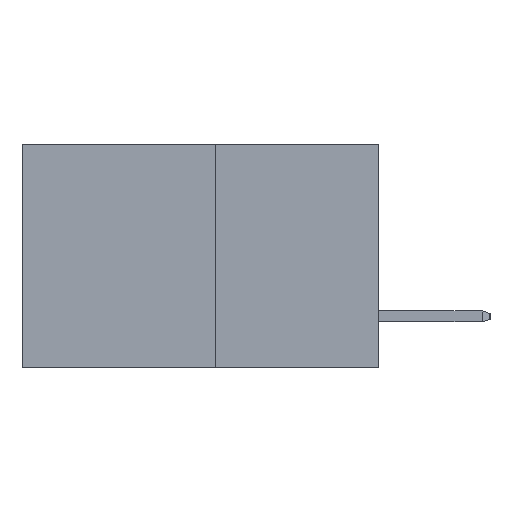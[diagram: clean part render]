
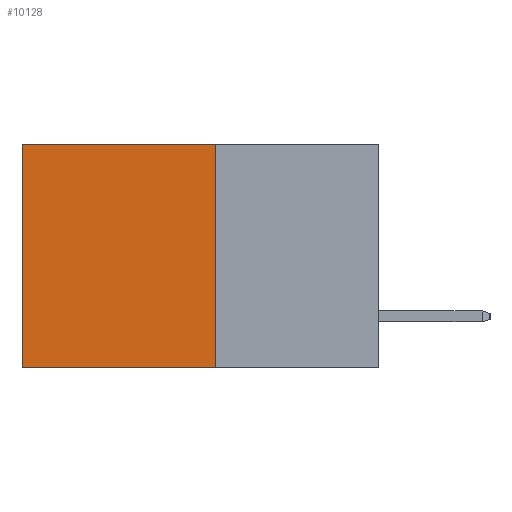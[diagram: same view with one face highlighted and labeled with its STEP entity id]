
A CAD part, left-side view. The second image highlights one B-rep face of the part: STEP entity #10128.
In plain terms, the highlighted planar face has unit normal (-1, 0, 0).
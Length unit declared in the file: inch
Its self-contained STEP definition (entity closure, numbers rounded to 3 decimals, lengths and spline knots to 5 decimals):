
#259 = ORIENTED_EDGE ( 'NONE', *, *, #10974, .T. ) ;
#437 = DIRECTION ( 'NONE',  ( 1., 0., 0. ) ) ;
#1027 = VERTEX_POINT ( 'NONE', #2424 ) ;
#1223 = ORIENTED_EDGE ( 'NONE', *, *, #10586, .F. ) ;
#1614 = ORIENTED_EDGE ( 'NONE', *, *, #4068, .F. ) ;
#2012 = VECTOR ( 'NONE', #6748, 39.37008 ) ;
#2424 = CARTESIAN_POINT ( 'NONE',  ( 0.277, 0.59, 0. ) ) ;
#2429 = CARTESIAN_POINT ( 'NONE',  ( 0.277, 0.59, -0.37 ) ) ;
#2477 = CARTESIAN_POINT ( 'NONE',  ( 0.277, 0.27, -0.37 ) ) ;
#3446 = LINE ( 'NONE', #11366, #6398 ) ;
#3470 = CARTESIAN_POINT ( 'NONE',  ( 0.277, 0.27, -0.37 ) ) ;
#3932 = DIRECTION ( 'NONE',  ( 0., 1., 0. ) ) ;
#3966 = ORIENTED_EDGE ( 'NONE', *, *, #10192, .T. ) ;
#4029 = AXIS2_PLACEMENT_3D ( 'NONE', #2477, #437, #7461 ) ;
#4068 = EDGE_CURVE ( 'NONE', #9602, #7658, #10323, .T. ) ;
#5152 = VERTEX_POINT ( 'NONE', #6351 ) ;
#5500 = VECTOR ( 'NONE', #3932, 39.37008 ) ;
#5583 = DIRECTION ( 'NONE',  ( 0., 1., 0. ) ) ;
#6221 = DIRECTION ( 'NONE',  ( 0., 0., -1. ) ) ;
#6351 = CARTESIAN_POINT ( 'NONE',  ( 0.277, 0.27, 0. ) ) ;
#6398 = VECTOR ( 'NONE', #5583, 39.37008 ) ;
#6480 = PLANE ( 'NONE',  #4029 ) ;
#6498 = EDGE_LOOP ( 'NONE', ( #259, #1614, #1223, #3966 ) ) ;
#6692 = FACE_OUTER_BOUND ( 'NONE', #6498, .T. ) ;
#6748 = DIRECTION ( 'NONE',  ( 0., 0., -1. ) ) ;
#7461 = DIRECTION ( 'NONE',  ( 0., 0., -1. ) ) ;
#7658 = VERTEX_POINT ( 'NONE', #2429 ) ;
#8999 = VECTOR ( 'NONE', #6221, 39.37008 ) ;
#9548 = LINE ( 'NONE', #12485, #2012 ) ;
#9602 = VERTEX_POINT ( 'NONE', #11458 ) ;
#10050 = CARTESIAN_POINT ( 'NONE',  ( 0.277, 0.27, -0.37 ) ) ;
#10128 = ADVANCED_FACE ( 'NONE', ( #6692 ), #6480, .F. ) ;
#10192 = EDGE_CURVE ( 'NONE', #5152, #1027, #3446, .T. ) ;
#10323 = LINE ( 'NONE', #3470, #5500 ) ;
#10586 = EDGE_CURVE ( 'NONE', #5152, #9602, #11505, .T. ) ;
#10974 = EDGE_CURVE ( 'NONE', #1027, #7658, #9548, .T. ) ;
#11366 = CARTESIAN_POINT ( 'NONE',  ( 0.277, 0.27, 0. ) ) ;
#11458 = CARTESIAN_POINT ( 'NONE',  ( 0.277, 0.27, -0.37 ) ) ;
#11505 = LINE ( 'NONE', #10050, #8999 ) ;
#12485 = CARTESIAN_POINT ( 'NONE',  ( 0.277, 0.59, -0.37 ) ) ;
